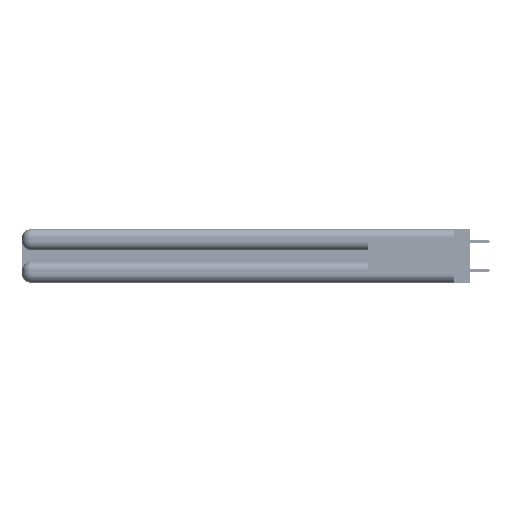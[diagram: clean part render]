
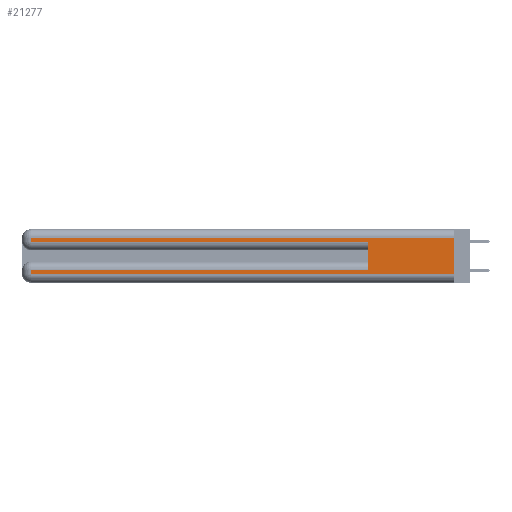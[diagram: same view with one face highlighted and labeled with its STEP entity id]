
A CAD part, left-side view. The second image highlights one B-rep face of the part: STEP entity #21277.
In plain terms, the highlighted planar face has unit normal (-1, 0, 0).
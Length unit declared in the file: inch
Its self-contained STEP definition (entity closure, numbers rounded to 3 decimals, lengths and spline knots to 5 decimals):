
#146 = DIRECTION ( 'NONE',  ( 1., 0., 0. ) ) ;
#1117 = LINE ( 'NONE', #33656, #14561 ) ;
#2332 = CARTESIAN_POINT ( 'NONE',  ( 0., 2.94, 0.37 ) ) ;
#2524 = ORIENTED_EDGE ( 'NONE', *, *, #3040, .T. ) ;
#3040 = EDGE_CURVE ( 'NONE', #23929, #11152, #6070, .T. ) ;
#4936 = LINE ( 'NONE', #34702, #17764 ) ;
#5176 = ORIENTED_EDGE ( 'NONE', *, *, #46619, .F. ) ;
#6070 = LINE ( 'NONE', #34493, #49611 ) ;
#6829 = CARTESIAN_POINT ( 'NONE',  ( 0., 2.94, 0.31 ) ) ;
#8018 = AXIS2_PLACEMENT_3D ( 'NONE', #29909, #146, #12716 ) ;
#9472 = VECTOR ( 'NONE', #9581, 39.37008 ) ;
#9581 = DIRECTION ( 'NONE',  ( 0., 0., -1. ) ) ;
#9942 = VECTOR ( 'NONE', #43159, 39.37008 ) ;
#11152 = VERTEX_POINT ( 'NONE', #28321 ) ;
#12716 = DIRECTION ( 'NONE',  ( 0., 0., -1. ) ) ;
#13321 = EDGE_CURVE ( 'NONE', #11152, #47631, #30336, .T. ) ;
#13686 = ORIENTED_EDGE ( 'NONE', *, *, #22949, .T. ) ;
#14561 = VECTOR ( 'NONE', #34187, 39.37008 ) ;
#15124 = VERTEX_POINT ( 'NONE', #16168 ) ;
#16168 = CARTESIAN_POINT ( 'NONE',  ( 0., 0., 0.06 ) ) ;
#17764 = VECTOR ( 'NONE', #34160, 39.37008 ) ;
#20911 = FACE_OUTER_BOUND ( 'NONE', #38370, .T. ) ;
#21277 = ADVANCED_FACE ( 'NONE', ( #20911 ), #46057, .F. ) ;
#21630 = CARTESIAN_POINT ( 'NONE',  ( 0., 2.94, 0.285 ) ) ;
#22087 = VECTOR ( 'NONE', #34814, 39.37008 ) ;
#22949 = EDGE_CURVE ( 'NONE', #47631, #15124, #45195, .T. ) ;
#23929 = VERTEX_POINT ( 'NONE', #25414 ) ;
#24714 = ORIENTED_EDGE ( 'NONE', *, *, #52571, .T. ) ;
#25414 = CARTESIAN_POINT ( 'NONE',  ( 0., 0.6, 0.085 ) ) ;
#26823 = CARTESIAN_POINT ( 'NONE',  ( 0., 0., 0.31 ) ) ;
#28218 = ORIENTED_EDGE ( 'NONE', *, *, #13321, .T. ) ;
#28321 = CARTESIAN_POINT ( 'NONE',  ( 0., 2.94, 0.085 ) ) ;
#29052 = DIRECTION ( 'NONE',  ( 0., -1., 0. ) ) ;
#29891 = LINE ( 'NONE', #38906, #22087 ) ;
#29909 = CARTESIAN_POINT ( 'NONE',  ( 0., 0., 0.37 ) ) ;
#30336 = LINE ( 'NONE', #43167, #9472 ) ;
#30574 = VERTEX_POINT ( 'NONE', #21630 ) ;
#30586 = LINE ( 'NONE', #50571, #9942 ) ;
#31543 = VECTOR ( 'NONE', #29052, 39.37008 ) ;
#33656 = CARTESIAN_POINT ( 'NONE',  ( 0., 0., 0.37 ) ) ;
#33692 = CARTESIAN_POINT ( 'NONE',  ( 0., 0.6, 0.285 ) ) ;
#34160 = DIRECTION ( 'NONE',  ( 0., 1., 0. ) ) ;
#34187 = DIRECTION ( 'NONE',  ( 0., 0., -1. ) ) ;
#34286 = EDGE_CURVE ( 'NONE', #41762, #48119, #4936, .T. ) ;
#34493 = CARTESIAN_POINT ( 'NONE',  ( 0., 0., 0.085 ) ) ;
#34702 = CARTESIAN_POINT ( 'NONE',  ( 0., 0., 0.31 ) ) ;
#34782 = ORIENTED_EDGE ( 'NONE', *, *, #39981, .T. ) ;
#34814 = DIRECTION ( 'NONE',  ( 0., -1., 0. ) ) ;
#37000 = CARTESIAN_POINT ( 'NONE',  ( 0., 0., 0.06 ) ) ;
#37694 = EDGE_CURVE ( 'NONE', #41762, #15124, #1117, .T. ) ;
#38370 = EDGE_LOOP ( 'NONE', ( #41923, #41300, #34782, #24714, #5176, #2524, #28218, #13686 ) ) ;
#38906 = CARTESIAN_POINT ( 'NONE',  ( 0., 0., 0.285 ) ) ;
#38967 = DIRECTION ( 'NONE',  ( 0., 0., -1. ) ) ;
#39759 = LINE ( 'NONE', #2332, #49530 ) ;
#39952 = CARTESIAN_POINT ( 'NONE',  ( 0., 2.94, 0.06 ) ) ;
#39981 = EDGE_CURVE ( 'NONE', #48119, #30574, #39759, .T. ) ;
#41300 = ORIENTED_EDGE ( 'NONE', *, *, #34286, .T. ) ;
#41762 = VERTEX_POINT ( 'NONE', #26823 ) ;
#41923 = ORIENTED_EDGE ( 'NONE', *, *, #37694, .F. ) ;
#42684 = DIRECTION ( 'NONE',  ( 0., 1., 0. ) ) ;
#42726 = VERTEX_POINT ( 'NONE', #33692 ) ;
#43159 = DIRECTION ( 'NONE',  ( 0., 0., 1. ) ) ;
#43167 = CARTESIAN_POINT ( 'NONE',  ( 0., 2.94, 0.37 ) ) ;
#45195 = LINE ( 'NONE', #37000, #31543 ) ;
#46057 = PLANE ( 'NONE',  #8018 ) ;
#46619 = EDGE_CURVE ( 'NONE', #23929, #42726, #30586, .T. ) ;
#47631 = VERTEX_POINT ( 'NONE', #39952 ) ;
#48119 = VERTEX_POINT ( 'NONE', #6829 ) ;
#49530 = VECTOR ( 'NONE', #38967, 39.37008 ) ;
#49611 = VECTOR ( 'NONE', #42684, 39.37008 ) ;
#50571 = CARTESIAN_POINT ( 'NONE',  ( 0., 0.6, 0.145 ) ) ;
#52571 = EDGE_CURVE ( 'NONE', #30574, #42726, #29891, .T. ) ;
